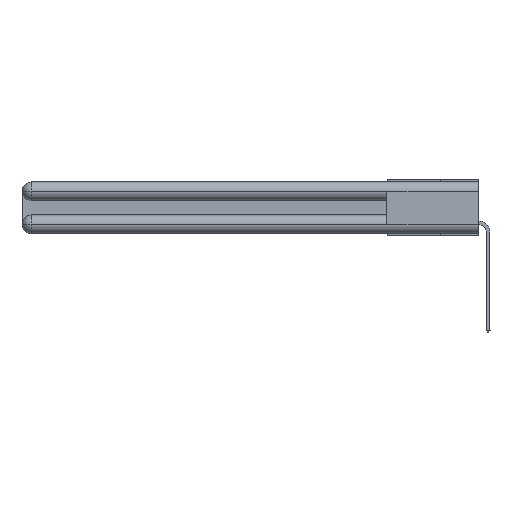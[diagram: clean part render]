
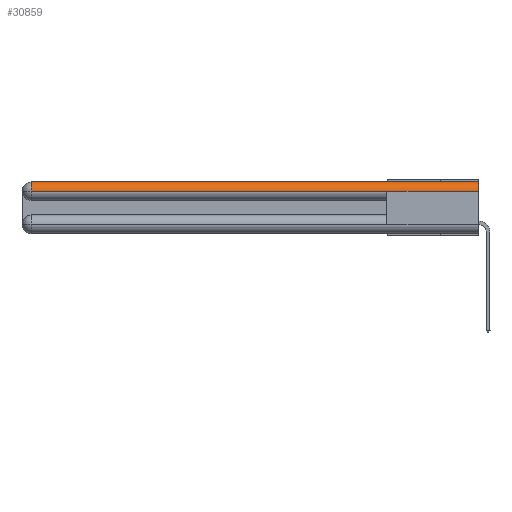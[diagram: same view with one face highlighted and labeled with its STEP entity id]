
A CAD part, left-side view. The second image highlights one B-rep face of the part: STEP entity #30859.
In plain terms, the highlighted cylindrical face has radius 1.562 mm (diameter 3.124 mm), a partial arc.
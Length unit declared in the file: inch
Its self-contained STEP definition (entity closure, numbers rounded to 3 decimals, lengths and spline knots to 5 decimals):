
#156 = VERTEX_POINT ( 'NONE', #26464 ) ;
#499 = EDGE_CURVE ( 'NONE', #18532, #12231, #29397, .T. ) ;
#2843 = CIRCLE ( 'NONE', #23999, 0.0615 ) ;
#3635 = DIRECTION ( 'NONE',  ( 0., 1., 0. ) ) ;
#3746 = CARTESIAN_POINT ( 'NONE',  ( 0.0615, 0., -0.0615 ) ) ;
#3772 = CARTESIAN_POINT ( 'NONE',  ( 0., 3., -0.0615 ) ) ;
#3985 = DIRECTION ( 'NONE',  ( 0., 1., 0. ) ) ;
#4795 = DIRECTION ( 'NONE',  ( 1., 0., 0. ) ) ;
#5264 = CARTESIAN_POINT ( 'NONE',  ( 0.0615, 0., -0.0615 ) ) ;
#6509 = ORIENTED_EDGE ( 'NONE', *, *, #499, .T. ) ;
#6637 = EDGE_CURVE ( 'NONE', #7600, #12231, #6769, .T. ) ;
#6647 = ORIENTED_EDGE ( 'NONE', *, *, #26761, .F. ) ;
#6769 = LINE ( 'NONE', #11694, #22575 ) ;
#7600 = VERTEX_POINT ( 'NONE', #25787 ) ;
#8177 = EDGE_LOOP ( 'NONE', ( #29126, #16355, #6509, #21576, #6647 ) ) ;
#9058 = EDGE_CURVE ( 'NONE', #156, #18532, #26622, .T. ) ;
#9100 = DIRECTION ( 'NONE',  ( 0., 0., 1. ) ) ;
#9796 = VECTOR ( 'NONE', #13305, 39.37008 ) ;
#10194 = LINE ( 'NONE', #10773, #9796 ) ;
#10773 = CARTESIAN_POINT ( 'NONE',  ( 0.0615, 0., 0. ) ) ;
#11251 = CARTESIAN_POINT ( 'NONE',  ( 0., 0.6, -0.0615 ) ) ;
#11694 = CARTESIAN_POINT ( 'NONE',  ( 0., 3., -0.0615 ) ) ;
#11815 = DIRECTION ( 'NONE',  ( 0., -1., 0. ) ) ;
#12231 = VERTEX_POINT ( 'NONE', #11251 ) ;
#12843 = DIRECTION ( 'NONE',  ( 0., -1., 0. ) ) ;
#13026 = CARTESIAN_POINT ( 'NONE',  ( 0., 2.94, -0.0615 ) ) ;
#13305 = DIRECTION ( 'NONE',  ( 0., -1., 0. ) ) ;
#15758 = DIRECTION ( 'NONE',  ( 0., 0., 1. ) ) ;
#16355 = ORIENTED_EDGE ( 'NONE', *, *, #9058, .T. ) ;
#16766 = VERTEX_POINT ( 'NONE', #20234 ) ;
#18532 = VERTEX_POINT ( 'NONE', #13026 ) ;
#20234 = CARTESIAN_POINT ( 'NONE',  ( 0.0615, 0., 0. ) ) ;
#21576 = ORIENTED_EDGE ( 'NONE', *, *, #6637, .F. ) ;
#22575 = VECTOR ( 'NONE', #3985, 39.37008 ) ;
#23121 = FACE_OUTER_BOUND ( 'NONE', #8177, .T. ) ;
#23623 = DIRECTION ( 'NONE',  ( 0., -1., 0. ) ) ;
#23999 = AXIS2_PLACEMENT_3D ( 'NONE', #5264, #23623, #4795 ) ;
#25787 = CARTESIAN_POINT ( 'NONE',  ( 0., 0., -0.0615 ) ) ;
#26464 = CARTESIAN_POINT ( 'NONE',  ( 0.0615, 2.94, 0. ) ) ;
#26622 = CIRCLE ( 'NONE', #30815, 0.0615 ) ;
#26761 = EDGE_CURVE ( 'NONE', #16766, #7600, #2843, .T. ) ;
#28232 = AXIS2_PLACEMENT_3D ( 'NONE', #3746, #3635, #9100 ) ;
#28353 = EDGE_CURVE ( 'NONE', #156, #16766, #10194, .T. ) ;
#29126 = ORIENTED_EDGE ( 'NONE', *, *, #28353, .F. ) ;
#29397 = LINE ( 'NONE', #3772, #31496 ) ;
#30680 = CYLINDRICAL_SURFACE ( 'NONE', #28232, 0.0615 ) ;
#30815 = AXIS2_PLACEMENT_3D ( 'NONE', #31755, #12843, #15758 ) ;
#30859 = ADVANCED_FACE ( 'NONE', ( #23121 ), #30680, .T. ) ;
#31496 = VECTOR ( 'NONE', #11815, 39.37008 ) ;
#31755 = CARTESIAN_POINT ( 'NONE',  ( 0.0615, 2.94, -0.0615 ) ) ;
